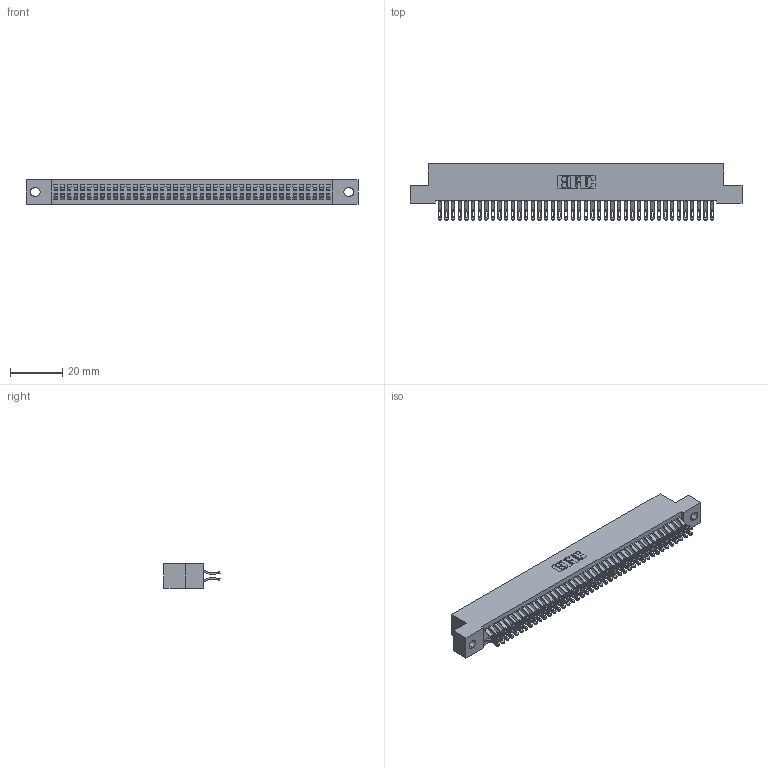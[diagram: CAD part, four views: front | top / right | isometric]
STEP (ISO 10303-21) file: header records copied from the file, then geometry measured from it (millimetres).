
FILE_DESCRIPTION (( 'STEP AP203' ), '1' );
FILE_NAME ('342-084-555-202.STEP', '2018-08-13T18:07:04', ( '' ), ( '' ), 'SwSTEP 2.0', 'SolidWorks 2016', '' );
FILE_SCHEMA (( 'CONFIG_CONTROL_DESIGN' ));
Length unit declared in the file: inch
Products named in the file (3): 345-292-001_555 Tail; 342-084-555-202; 342 Part_.128 Slot
Assembly tree (85 placements, depth 2):
  342-084-555-202
    342 Part_.128 Slot
    345-292-001_555 Tail  x84
Bounding box: 127 x 21.47 x 9.4 mm (x, y, z)
Volume: 11592.2 mm3; surface area: 19441.5 mm2
Topology: 85 solids, 85 shells, 4986 faces, 15683 edges, 10454 vertices
Faces by surface type: plane 2926, cylinder 2060
Entity records: 27349 total; most frequent: CARTESIAN_POINT 4568, ORIENTED_EDGE 4474, DIRECTION 3873, EDGE_CURVE 2237, LINE 2089, VECTOR 2089, VERTEX_POINT 1490, AXIS2_PLACEMENT_3D 892
